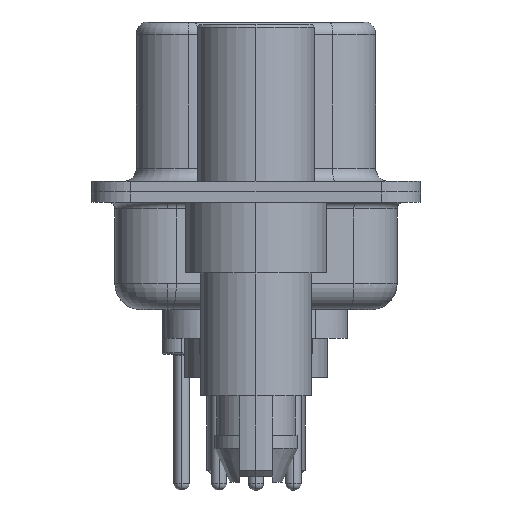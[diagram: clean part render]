
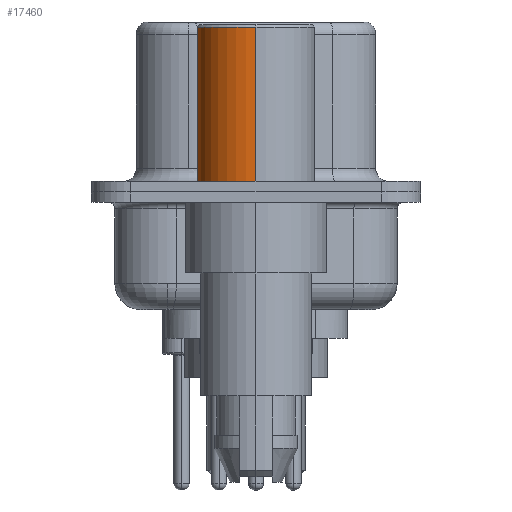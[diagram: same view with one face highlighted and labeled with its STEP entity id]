
A CAD part, left-side view. The second image highlights one B-rep face of the part: STEP entity #17460.
In plain terms, the highlighted cylindrical face has radius 2.25 mm (diameter 4.5 mm), a partial arc.
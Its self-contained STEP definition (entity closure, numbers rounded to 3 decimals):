
#779 = FACE_OUTER_BOUND ( 'NONE', #3240, .T. ) ;
#1106 = DIRECTION ( 'NONE',  ( 1., 0., 0. ) ) ;
#2336 = CIRCLE ( 'NONE', #15072, 2.25 ) ;
#3240 = EDGE_LOOP ( 'NONE', ( #23712, #10185, #17005, #23968 ) ) ;
#3790 = VERTEX_POINT ( 'NONE', #13446 ) ;
#4226 = DIRECTION ( 'NONE',  ( 1., 0., 0. ) ) ;
#5633 = LINE ( 'NONE', #21134, #15198 ) ;
#6617 = DIRECTION ( 'NONE',  ( 0., 0., 1. ) ) ;
#7399 = DIRECTION ( 'NONE',  ( 1., 0., 0. ) ) ;
#8212 = CARTESIAN_POINT ( 'NONE',  ( -2.25, 0., 6.3 ) ) ;
#8493 = DIRECTION ( 'NONE',  ( 0., 0., 1. ) ) ;
#10185 = ORIENTED_EDGE ( 'NONE', *, *, #19840, .T. ) ;
#10446 = AXIS2_PLACEMENT_3D ( 'NONE', #19820, #14308, #7399 ) ;
#11036 = CYLINDRICAL_SURFACE ( 'NONE', #10446, 2.25 ) ;
#11421 = VERTEX_POINT ( 'NONE', #18352 ) ;
#11994 = AXIS2_PLACEMENT_3D ( 'NONE', #12528, #15904, #4226 ) ;
#12382 = EDGE_CURVE ( 'NONE', #11421, #3790, #5633, .T. ) ;
#12392 = VERTEX_POINT ( 'NONE', #21208 ) ;
#12528 = CARTESIAN_POINT ( 'NONE',  ( 0., 0., 6.3 ) ) ;
#13446 = CARTESIAN_POINT ( 'NONE',  ( 2.25, 0., 6.3 ) ) ;
#14308 = DIRECTION ( 'NONE',  ( 0., 0., 1. ) ) ;
#15072 = AXIS2_PLACEMENT_3D ( 'NONE', #15918, #6617, #1106 ) ;
#15198 = VECTOR ( 'NONE', #8493, 1000. ) ;
#15904 = DIRECTION ( 'NONE',  ( 0., 0., 1. ) ) ;
#15918 = CARTESIAN_POINT ( 'NONE',  ( 0., 0., 0.4 ) ) ;
#17005 = ORIENTED_EDGE ( 'NONE', *, *, #21264, .F. ) ;
#17460 = ADVANCED_FACE ( 'NONE', ( #779 ), #11036, .T. ) ;
#17541 = CIRCLE ( 'NONE', #11994, 2.25 ) ;
#18352 = CARTESIAN_POINT ( 'NONE',  ( 2.25, 0., 0.4 ) ) ;
#19820 = CARTESIAN_POINT ( 'NONE',  ( 0., 0., 0.581 ) ) ;
#19840 = EDGE_CURVE ( 'NONE', #12392, #21624, #20795, .T. ) ;
#20795 = LINE ( 'NONE', #23116, #23978 ) ;
#21100 = DIRECTION ( 'NONE',  ( 0., 0., 1. ) ) ;
#21134 = CARTESIAN_POINT ( 'NONE',  ( 2.25, 0., 0.581 ) ) ;
#21208 = CARTESIAN_POINT ( 'NONE',  ( -2.25, 0., 0.4 ) ) ;
#21264 = EDGE_CURVE ( 'NONE', #3790, #21624, #17541, .T. ) ;
#21624 = VERTEX_POINT ( 'NONE', #8212 ) ;
#21761 = EDGE_CURVE ( 'NONE', #11421, #12392, #2336, .T. ) ;
#23116 = CARTESIAN_POINT ( 'NONE',  ( -2.25, 0., 0.581 ) ) ;
#23712 = ORIENTED_EDGE ( 'NONE', *, *, #21761, .T. ) ;
#23968 = ORIENTED_EDGE ( 'NONE', *, *, #12382, .F. ) ;
#23978 = VECTOR ( 'NONE', #21100, 1000. ) ;
